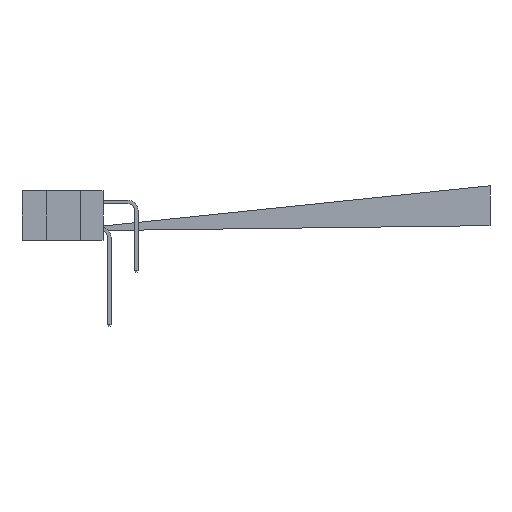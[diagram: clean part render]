
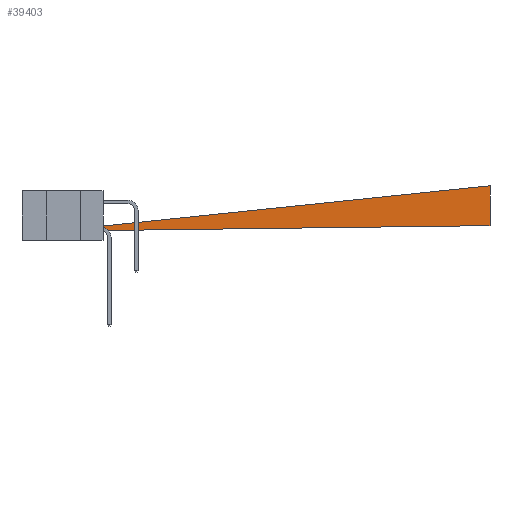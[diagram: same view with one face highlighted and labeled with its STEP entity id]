
A CAD part, left-side view. The second image highlights one B-rep face of the part: STEP entity #39403.
In plain terms, the highlighted face is planar.
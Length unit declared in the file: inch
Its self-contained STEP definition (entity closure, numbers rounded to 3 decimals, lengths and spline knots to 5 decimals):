
#219 = EDGE_CURVE ( 'NONE', #26266, #20639, #3180, .T. ) ;
#224 = EDGE_CURVE ( 'NONE', #5033, #34478, #23322, .T. ) ;
#832 = PLANE ( 'NONE',  #20102 ) ;
#1264 = EDGE_CURVE ( 'NONE', #11898, #25995, #37493, .T. ) ;
#3116 = CIRCLE ( 'NONE', #44385, 0.0185 ) ;
#3180 = CIRCLE ( 'NONE', #37761, 0.0765 ) ;
#3384 = CARTESIAN_POINT ( 'NONE',  ( 0.21268, 0.09924, -0.025 ) ) ;
#3463 = VERTEX_POINT ( 'NONE', #34166 ) ;
#3939 = VECTOR ( 'NONE', #46448, 39.37008 ) ;
#3957 = DIRECTION ( 'NONE',  ( 0., 0., -1. ) ) ;
#3962 = AXIS2_PLACEMENT_3D ( 'NONE', #37720, #9571, #20702 ) ;
#4439 = DIRECTION ( 'NONE',  ( 0., 0., -1. ) ) ;
#4614 = EDGE_CURVE ( 'NONE', #20639, #5033, #3116, .T. ) ;
#4815 = DIRECTION ( 'NONE',  ( 1., 0., 0. ) ) ;
#5033 = VERTEX_POINT ( 'NONE', #29907 ) ;
#5083 = CIRCLE ( 'NONE', #27309, 0.0135 ) ;
#5180 = CARTESIAN_POINT ( 'NONE',  ( 3.5375, 0.345, -0.0975 ) ) ;
#5253 = EDGE_CURVE ( 'NONE', #45232, #38249, #30107, .T. ) ;
#5469 = ORIENTED_EDGE ( 'NONE', *, *, #35809, .T. ) ;
#6186 = EDGE_CURVE ( 'NONE', #34478, #46514, #6620, .T. ) ;
#6275 = AXIS2_PLACEMENT_3D ( 'NONE', #30990, #8752, #34605 ) ;
#6279 = VERTEX_POINT ( 'NONE', #37405 ) ;
#6620 = CIRCLE ( 'NONE', #3962, 0.02173 ) ;
#7162 = VERTEX_POINT ( 'NONE', #43836 ) ;
#7348 = CARTESIAN_POINT ( 'NONE',  ( 0.33619, 0.0125, -0.025 ) ) ;
#7393 = DIRECTION ( 'NONE',  ( 1., 0., 0. ) ) ;
#7543 = CARTESIAN_POINT ( 'NONE',  ( 0.33619, 0.044, -0.025 ) ) ;
#8192 = DIRECTION ( 'NONE',  ( 1., 0., 0. ) ) ;
#8433 = ORIENTED_EDGE ( 'NONE', *, *, #44326, .T. ) ;
#8752 = DIRECTION ( 'NONE',  ( 0., 0., -1. ) ) ;
#9115 = EDGE_CURVE ( 'NONE', #6279, #26264, #25935, .T. ) ;
#9571 = DIRECTION ( 'NONE',  ( 0., 0., 1. ) ) ;
#11055 = ORIENTED_EDGE ( 'NONE', *, *, #25165, .F. ) ;
#11401 = DIRECTION ( 'NONE',  ( 1., 0., 0. ) ) ;
#11490 = DIRECTION ( 'NONE',  ( -1., 0., 0. ) ) ;
#11898 = VERTEX_POINT ( 'NONE', #14419 ) ;
#12553 = CARTESIAN_POINT ( 'NONE',  ( 0.33619, 0.0255, -0.025 ) ) ;
#13835 = ORIENTED_EDGE ( 'NONE', *, *, #6186, .T. ) ;
#14419 = CARTESIAN_POINT ( 'NONE',  ( 0.14622, 0.058, -0.025 ) ) ;
#16070 = CARTESIAN_POINT ( 'NONE',  ( 0.13321, 0.058, -0.025 ) ) ;
#16081 = CARTESIAN_POINT ( 'NONE',  ( 0.14781, 0.08118, -0.025 ) ) ;
#16642 = CARTESIAN_POINT ( 'NONE',  ( 0.58021, 0.0375, -0.025 ) ) ;
#17084 = CARTESIAN_POINT ( 'NONE',  ( 0.45821, 0.0375, -0.025 ) ) ;
#18098 = EDGE_CURVE ( 'NONE', #46514, #45232, #18511, .T. ) ;
#18511 = LINE ( 'NONE', #34474, #37989 ) ;
#19152 = VECTOR ( 'NONE', #8192, 39.37008 ) ;
#19959 = AXIS2_PLACEMENT_3D ( 'NONE', #26959, #4439, #30662 ) ;
#19979 = DIRECTION ( 'NONE',  ( 0.893, 0.449, 0. ) ) ;
#19983 = VERTEX_POINT ( 'NONE', #5180 ) ;
#20102 = AXIS2_PLACEMENT_3D ( 'NONE', #23599, #27322, #4815 ) ;
#20639 = VERTEX_POINT ( 'NONE', #40139 ) ;
#20682 = ORIENTED_EDGE ( 'NONE', *, *, #5469, .F. ) ;
#20702 = DIRECTION ( 'NONE',  ( 1., 0., 0. ) ) ;
#21302 = LINE ( 'NONE', #16642, #48208 ) ;
#21823 = AXIS2_PLACEMENT_3D ( 'NONE', #7543, #33496, #11401 ) ;
#22184 = CARTESIAN_POINT ( 'NONE',  ( 3.5375, 0.05, -0.0975 ) ) ;
#23322 = LINE ( 'NONE', #12553, #47939 ) ;
#23599 = CARTESIAN_POINT ( 'NONE',  ( 0.095, 0.025, -0.025 ) ) ;
#24099 = CARTESIAN_POINT ( 'NONE',  ( 0.33619, 0.0125, -0.025 ) ) ;
#25165 = EDGE_CURVE ( 'NONE', #26264, #3463, #41783, .T. ) ;
#25352 = ORIENTED_EDGE ( 'NONE', *, *, #224, .T. ) ;
#25935 = CIRCLE ( 'NONE', #21823, 0.0315 ) ;
#25995 = VERTEX_POINT ( 'NONE', #45936 ) ;
#26264 = VERTEX_POINT ( 'NONE', #7348 ) ;
#26266 = VERTEX_POINT ( 'NONE', #33309 ) ;
#26395 = ORIENTED_EDGE ( 'NONE', *, *, #34295, .F. ) ;
#26407 = DIRECTION ( 'NONE',  ( 0., 0., 1. ) ) ;
#26508 = CARTESIAN_POINT ( 'NONE',  ( 0.15971, 0.0575, -0.025 ) ) ;
#26657 = VECTOR ( 'NONE', #28649, 39.37008 ) ;
#26959 = CARTESIAN_POINT ( 'NONE',  ( 0.2412, 0.0425, -0.025 ) ) ;
#27214 = FACE_OUTER_BOUND ( 'NONE', #32676, .T. ) ;
#27309 = AXIS2_PLACEMENT_3D ( 'NONE', #26508, #3957, #30221 ) ;
#27322 = DIRECTION ( 'NONE',  ( 0., 0., 1. ) ) ;
#28649 = DIRECTION ( 'NONE',  ( -1., 0., 0. ) ) ;
#29065 = ORIENTED_EDGE ( 'NONE', *, *, #219, .T. ) ;
#29907 = CARTESIAN_POINT ( 'NONE',  ( 0.33619, 0.0255, -0.025 ) ) ;
#30107 = LINE ( 'NONE', #40063, #19152 ) ;
#30221 = DIRECTION ( 'NONE',  ( -1., 0., 0. ) ) ;
#30223 = CARTESIAN_POINT ( 'NONE',  ( 0.33619, 0.044, -0.025 ) ) ;
#30662 = DIRECTION ( 'NONE',  ( -1., 0., 0. ) ) ;
#30876 = VERTEX_POINT ( 'NONE', #35930 ) ;
#30990 = CARTESIAN_POINT ( 'NONE',  ( 0.15971, 0.0575, -0.025 ) ) ;
#31347 = EDGE_CURVE ( 'NONE', #38249, #3463, #21302, .T. ) ;
#31665 = ORIENTED_EDGE ( 'NONE', *, *, #31347, .T. ) ;
#32259 = VECTOR ( 'NONE', #19979, 39.37008 ) ;
#32676 = EDGE_LOOP ( 'NONE', ( #44800, #32809, #8433, #46509, #29065, #35153, #25352, #13835, #39361, #41073, #31665, #11055, #45152, #26395, #20682 ) ) ;
#32809 = ORIENTED_EDGE ( 'NONE', *, *, #1264, .T. ) ;
#33309 = CARTESIAN_POINT ( 'NONE',  ( 0.20684, 0.11085, -0.025 ) ) ;
#33496 = DIRECTION ( 'NONE',  ( 0., 0., 1. ) ) ;
#34166 = CARTESIAN_POINT ( 'NONE',  ( 0.58021, 0.0125, -0.025 ) ) ;
#34295 = EDGE_CURVE ( 'NONE', #44819, #6279, #36165, .T. ) ;
#34474 = CARTESIAN_POINT ( 'NONE',  ( 0.45821, 0.0375, -0.025 ) ) ;
#34478 = VERTEX_POINT ( 'NONE', #38881 ) ;
#34605 = DIRECTION ( 'NONE',  ( -1., 0., 0. ) ) ;
#34847 = LINE ( 'NONE', #42800, #3939 ) ;
#34899 = CARTESIAN_POINT ( 'NONE',  ( 0.45258, 0.03186, -0.025 ) ) ;
#35153 = ORIENTED_EDGE ( 'NONE', *, *, #4614, .T. ) ;
#35809 = EDGE_CURVE ( 'NONE', #39066, #19983, #34847, .T. ) ;
#35930 = CARTESIAN_POINT ( 'NONE',  ( 0.14781, 0.08118, -0.025 ) ) ;
#36165 = CIRCLE ( 'NONE', #19959, 0.0635 ) ;
#36888 = CARTESIAN_POINT ( 'NONE',  ( 0.2412, 0.0425, -0.025 ) ) ;
#37405 = CARTESIAN_POINT ( 'NONE',  ( 0.30469, 0.0435, -0.025 ) ) ;
#37493 = LINE ( 'NONE', #16070, #26657 ) ;
#37651 = CIRCLE ( 'NONE', #6275, 0.0265 ) ;
#37720 = CARTESIAN_POINT ( 'NONE',  ( 0.43721, 0.04723, -0.025 ) ) ;
#37761 = AXIS2_PLACEMENT_3D ( 'NONE', #36888, #45129, #11490 ) ;
#37989 = VECTOR ( 'NONE', #38000, 39.37008 ) ;
#38000 = DIRECTION ( 'NONE',  ( 0.707, 0.707, 0. ) ) ;
#38249 = VERTEX_POINT ( 'NONE', #47036 ) ;
#38772 = DIRECTION ( 'NONE',  ( 0., -1., 0. ) ) ;
#38881 = CARTESIAN_POINT ( 'NONE',  ( 0.43721, 0.0255, -0.025 ) ) ;
#39066 = VERTEX_POINT ( 'NONE', #22184 ) ;
#39361 = ORIENTED_EDGE ( 'NONE', *, *, #18098, .T. ) ;
#39403 = ADVANCED_FACE ( 'NONE', ( #27214 ), #832, .F. ) ;
#39486 = VECTOR ( 'NONE', #45999, 39.37008 ) ;
#40063 = CARTESIAN_POINT ( 'NONE',  ( 0.45821, 0.0375, -0.025 ) ) ;
#40139 = CARTESIAN_POINT ( 'NONE',  ( 0.31769, 0.04371, -0.025 ) ) ;
#41073 = ORIENTED_EDGE ( 'NONE', *, *, #5253, .T. ) ;
#41460 = DIRECTION ( 'NONE',  ( 1., 0., 0. ) ) ;
#41783 = LINE ( 'NONE', #24099, #39486 ) ;
#41946 = LINE ( 'NONE', #16081, #32259 ) ;
#42800 = CARTESIAN_POINT ( 'NONE',  ( 3.5375, 0.345, -0.0975 ) ) ;
#43836 = CARTESIAN_POINT ( 'NONE',  ( 0.15365, 0.06956, -0.025 ) ) ;
#44114 = EDGE_CURVE ( 'NONE', #11898, #7162, #5083, .T. ) ;
#44326 = EDGE_CURVE ( 'NONE', #25995, #30876, #37651, .T. ) ;
#44385 = AXIS2_PLACEMENT_3D ( 'NONE', #30223, #26407, #41460 ) ;
#44800 = ORIENTED_EDGE ( 'NONE', *, *, #44114, .F. ) ;
#44819 = VERTEX_POINT ( 'NONE', #3384 ) ;
#45129 = DIRECTION ( 'NONE',  ( 0., 0., -1. ) ) ;
#45152 = ORIENTED_EDGE ( 'NONE', *, *, #9115, .F. ) ;
#45232 = VERTEX_POINT ( 'NONE', #17084 ) ;
#45936 = CARTESIAN_POINT ( 'NONE',  ( 0.13322, 0.058, -0.025 ) ) ;
#45999 = DIRECTION ( 'NONE',  ( 1., 0., 0. ) ) ;
#46448 = DIRECTION ( 'NONE',  ( 0., 1., 0. ) ) ;
#46509 = ORIENTED_EDGE ( 'NONE', *, *, #47781, .T. ) ;
#46514 = VERTEX_POINT ( 'NONE', #34899 ) ;
#47036 = CARTESIAN_POINT ( 'NONE',  ( 0.58021, 0.0375, -0.025 ) ) ;
#47781 = EDGE_CURVE ( 'NONE', #30876, #26266, #41946, .T. ) ;
#47939 = VECTOR ( 'NONE', #7393, 39.37008 ) ;
#48208 = VECTOR ( 'NONE', #38772, 39.37008 ) ;
